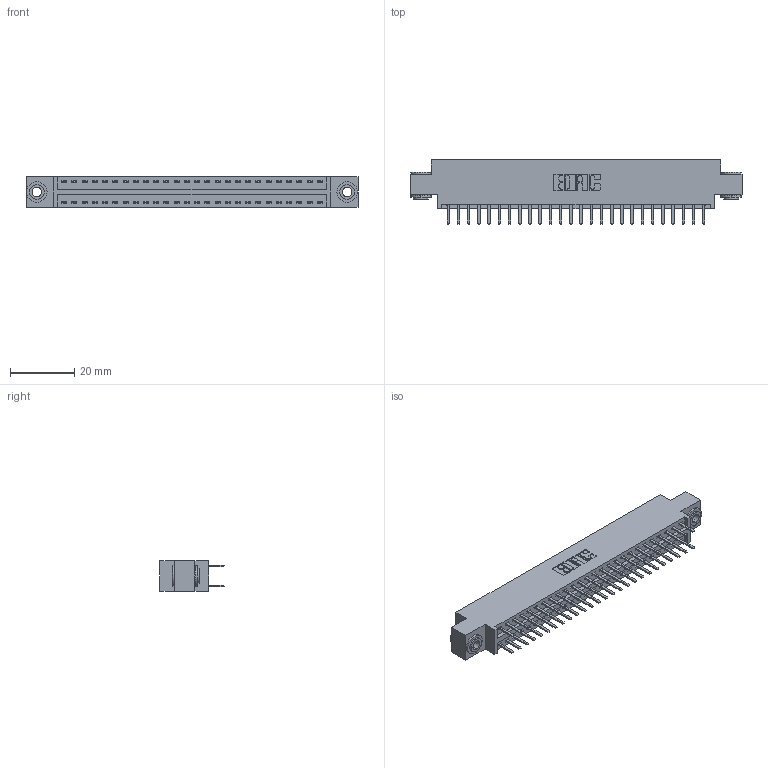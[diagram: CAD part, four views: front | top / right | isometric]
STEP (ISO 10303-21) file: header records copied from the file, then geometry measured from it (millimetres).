
FILE_DESCRIPTION (( 'STEP AP203' ), '1' );
FILE_NAME ('346-052-520-803.STEP', '2022-05-21T00:37:38', ( '' ), ( '' ), 'SwSTEP 2.0', 'SolidWorks 2020', '' );
FILE_SCHEMA (( 'CONFIG_CONTROL_DESIGN' ));
Length unit declared in the file: inch
Products named in the file (4): 346 Part_0.170 Offset - 0.156 Dia-TH; 345-292-001_345-293-120; 345-250-002_345-250-002-102; 346-052-520-803
Assembly tree (55 placements, depth 2):
  346-052-520-803
    346 Part_0.170 Offset - 0.156 Dia-TH
    345-292-001_345-293-120  x52
    345-250-002_345-250-002-102  x2
Bounding box: 103.12 x 20.02 x 9.4 mm (x, y, z)
Volume: 9755.4 mm3; surface area: 13532.8 mm2
Topology: 55 solids, 55 shells, 3090 faces, 8929 edges, 5810 vertices
Faces by surface type: plane 2028, cylinder 1054, cone 8
Entity records: 20434 total; most frequent: CARTESIAN_POINT 3385, ORIENTED_EDGE 3298, DIRECTION 3051, EDGE_CURVE 1649, VECTOR 1385, LINE 1385, VERTEX_POINT 1094, AXIS2_PLACEMENT_3D 833
